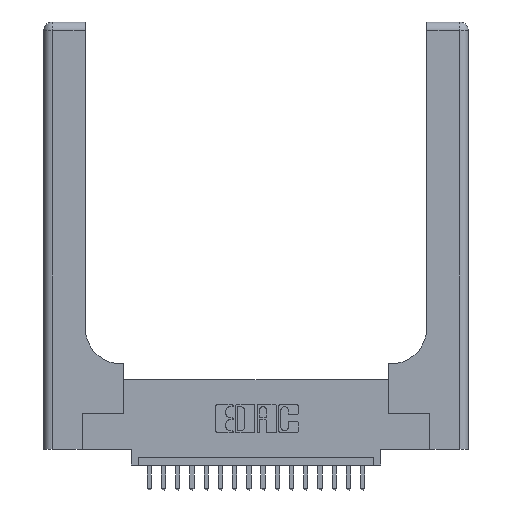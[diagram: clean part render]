
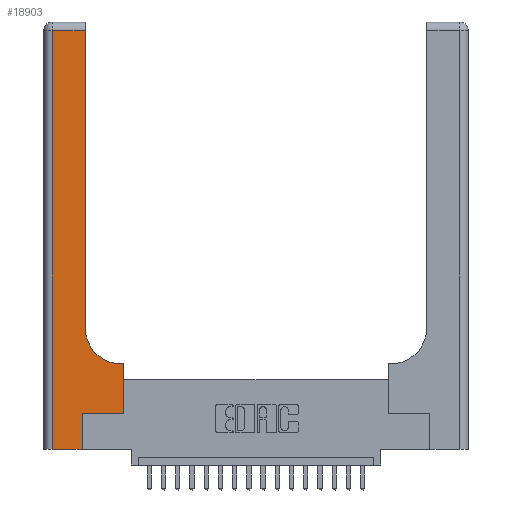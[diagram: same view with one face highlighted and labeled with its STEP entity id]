
A CAD part, top view. The second image highlights one B-rep face of the part: STEP entity #18903.
In plain terms, the highlighted planar face has unit normal (0, 0, 1).
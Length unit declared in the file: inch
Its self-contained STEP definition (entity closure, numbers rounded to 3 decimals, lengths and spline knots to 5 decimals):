
#926 = EDGE_CURVE ( 'NONE', #18494, #5132, #17653, .T. ) ;
#1590 = LINE ( 'NONE', #9813, #12998 ) ;
#1693 = CARTESIAN_POINT ( 'NONE',  ( 0.06, 0., 0.37 ) ) ;
#1859 = CARTESIAN_POINT ( 'NONE',  ( 0.2915, 3., 0.37 ) ) ;
#1954 = EDGE_CURVE ( 'NONE', #13239, #4031, #7731, .T. ) ;
#1963 = DIRECTION ( 'NONE',  ( -1., 0., 0. ) ) ;
#2047 = CARTESIAN_POINT ( 'NONE',  ( 0.269, 0., 0.37 ) ) ;
#2370 = EDGE_CURVE ( 'NONE', #18424, #2845, #2383, .T. ) ;
#2383 = LINE ( 'NONE', #19089, #9006 ) ;
#2391 = LINE ( 'NONE', #11447, #6948 ) ;
#2845 = VERTEX_POINT ( 'NONE', #10875 ) ;
#3124 = VERTEX_POINT ( 'NONE', #9545 ) ;
#3518 = DIRECTION ( 'NONE',  ( 0., 0., -1. ) ) ;
#3606 = DIRECTION ( 'NONE',  ( 0., -1., 0. ) ) ;
#3740 = CIRCLE ( 'NONE', #6475, 0.25 ) ;
#3917 = CARTESIAN_POINT ( 'NONE',  ( 0.06, 2.94, 0.37 ) ) ;
#4031 = VERTEX_POINT ( 'NONE', #5803 ) ;
#4339 = VERTEX_POINT ( 'NONE', #1693 ) ;
#4989 = VECTOR ( 'NONE', #8459, 39.37008 ) ;
#5132 = VERTEX_POINT ( 'NONE', #3917 ) ;
#5371 = ORIENTED_EDGE ( 'NONE', *, *, #9716, .T. ) ;
#5425 = EDGE_CURVE ( 'NONE', #4031, #3124, #18467, .T. ) ;
#5599 = CARTESIAN_POINT ( 'NONE',  ( 0., 0., 0.37 ) ) ;
#5803 = CARTESIAN_POINT ( 'NONE',  ( 0.269, 0.25, 0.37 ) ) ;
#5842 = CARTESIAN_POINT ( 'NONE',  ( 0.269, 0., 0.37 ) ) ;
#6431 = CARTESIAN_POINT ( 'NONE',  ( 0.5585, 0.6, 0.37 ) ) ;
#6475 = AXIS2_PLACEMENT_3D ( 'NONE', #19956, #3518, #13305 ) ;
#6579 = CARTESIAN_POINT ( 'NONE',  ( 0.2915, 2.94, 0.37 ) ) ;
#6929 = EDGE_CURVE ( 'NONE', #13479, #18494, #8295, .T. ) ;
#6948 = VECTOR ( 'NONE', #3606, 39.37008 ) ;
#7468 = DIRECTION ( 'NONE',  ( -1., 0., 0. ) ) ;
#7716 = DIRECTION ( 'NONE',  ( 0., 1., 0. ) ) ;
#7731 = LINE ( 'NONE', #5842, #10804 ) ;
#7918 = DIRECTION ( 'NONE',  ( 0., 1., 0. ) ) ;
#8295 = LINE ( 'NONE', #1859, #4989 ) ;
#8459 = DIRECTION ( 'NONE',  ( 0., 1., 0. ) ) ;
#9006 = VECTOR ( 'NONE', #9195, 39.37008 ) ;
#9195 = DIRECTION ( 'NONE',  ( -1., 0., 0. ) ) ;
#9545 = CARTESIAN_POINT ( 'NONE',  ( 0.5585, 0.25, 0.37 ) ) ;
#9553 = VECTOR ( 'NONE', #7468, 39.37008 ) ;
#9653 = EDGE_CURVE ( 'NONE', #5132, #4339, #2391, .T. ) ;
#9716 = EDGE_CURVE ( 'NONE', #4339, #13239, #14826, .T. ) ;
#9742 = ORIENTED_EDGE ( 'NONE', *, *, #1954, .T. ) ;
#9813 = CARTESIAN_POINT ( 'NONE',  ( 0.5585, 0.25, 0.37 ) ) ;
#10024 = CARTESIAN_POINT ( 'NONE',  ( 0., 3., 0.37 ) ) ;
#10128 = FACE_OUTER_BOUND ( 'NONE', #19972, .T. ) ;
#10804 = VECTOR ( 'NONE', #7918, 39.37008 ) ;
#10875 = CARTESIAN_POINT ( 'NONE',  ( 0.5415, 0.6, 0.37 ) ) ;
#11332 = ORIENTED_EDGE ( 'NONE', *, *, #13816, .T. ) ;
#11447 = CARTESIAN_POINT ( 'NONE',  ( 0.06, 3., 0.37 ) ) ;
#11702 = DIRECTION ( 'NONE',  ( 0., 0., -1. ) ) ;
#12998 = VECTOR ( 'NONE', #7716, 39.37008 ) ;
#13120 = ORIENTED_EDGE ( 'NONE', *, *, #926, .T. ) ;
#13239 = VERTEX_POINT ( 'NONE', #2047 ) ;
#13305 = DIRECTION ( 'NONE',  ( 1., 0., 0. ) ) ;
#13479 = VERTEX_POINT ( 'NONE', #15519 ) ;
#13816 = EDGE_CURVE ( 'NONE', #2845, #13479, #3740, .T. ) ;
#13970 = ORIENTED_EDGE ( 'NONE', *, *, #9653, .T. ) ;
#14151 = VECTOR ( 'NONE', #14687, 39.37008 ) ;
#14687 = DIRECTION ( 'NONE',  ( 1., 0., 0. ) ) ;
#14826 = LINE ( 'NONE', #5599, #18128 ) ;
#15017 = PLANE ( 'NONE',  #15507 ) ;
#15090 = DIRECTION ( 'NONE',  ( 1., 0., 0. ) ) ;
#15507 = AXIS2_PLACEMENT_3D ( 'NONE', #10024, #11702, #1963 ) ;
#15519 = CARTESIAN_POINT ( 'NONE',  ( 0.2915, 0.85, 0.37 ) ) ;
#15811 = ORIENTED_EDGE ( 'NONE', *, *, #2370, .T. ) ;
#15889 = ORIENTED_EDGE ( 'NONE', *, *, #5425, .T. ) ;
#15939 = EDGE_CURVE ( 'NONE', #3124, #18424, #1590, .T. ) ;
#17653 = LINE ( 'NONE', #18945, #9553 ) ;
#18128 = VECTOR ( 'NONE', #15090, 39.37008 ) ;
#18424 = VERTEX_POINT ( 'NONE', #6431 ) ;
#18467 = LINE ( 'NONE', #19427, #14151 ) ;
#18494 = VERTEX_POINT ( 'NONE', #6579 ) ;
#18868 = ORIENTED_EDGE ( 'NONE', *, *, #15939, .T. ) ;
#18903 = ADVANCED_FACE ( 'NONE', ( #10128 ), #15017, .F. ) ;
#18945 = CARTESIAN_POINT ( 'NONE',  ( 0., 2.94, 0.37 ) ) ;
#19089 = CARTESIAN_POINT ( 'NONE',  ( 0.2915, 0.6, 0.37 ) ) ;
#19427 = CARTESIAN_POINT ( 'NONE',  ( 0.269, 0.25, 0.37 ) ) ;
#19956 = CARTESIAN_POINT ( 'NONE',  ( 0.5415, 0.85, 0.37 ) ) ;
#19972 = EDGE_LOOP ( 'NONE', ( #20170, #13120, #13970, #5371, #9742, #15889, #18868, #15811, #11332 ) ) ;
#20170 = ORIENTED_EDGE ( 'NONE', *, *, #6929, .T. ) ;
